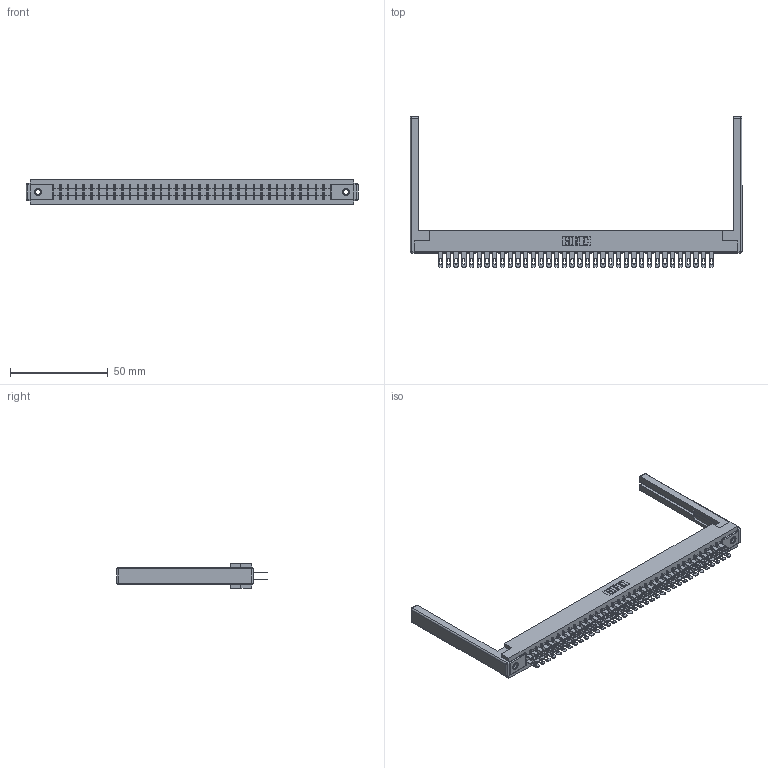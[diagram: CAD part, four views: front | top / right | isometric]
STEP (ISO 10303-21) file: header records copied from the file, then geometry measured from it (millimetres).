
FILE_DESCRIPTION (( 'STEP AP203' ), '1' );
FILE_NAME ('355-072-500-568.STEP', '2019-09-12T17:55:40', ( '' ), ( '' ), 'SwSTEP 2.0', 'SolidWorks 2016', '' );
FILE_SCHEMA (( 'CONFIG_CONTROL_DESIGN' ));
Length unit declared in the file: inch
Products named in the file (5): 307-220-068; 355-072-500-568; 305 Part_.156 Dia; 345-250-001_345-250-001-102; 305-290-001_500
Assembly tree (77 placements, depth 2):
  355-072-500-568
    305 Part_.156 Dia
    305-290-001_500  x72
    345-250-001_345-250-001-102  x2
    307-220-068  x2
Bounding box: 170.08 x 77.14 x 12.7 mm (x, y, z)
Volume: 21821.1 mm3; surface area: 28217.7 mm2
Topology: 77 solids, 77 shells, 3870 faces, 11038 edges, 7144 vertices
Faces by surface type: plane 2172, cylinder 1530, sphere 152, cone 12, torus 4
Entity records: 42490 total; most frequent: CARTESIAN_POINT 7003, ORIENTED_EDGE 6942, DIRECTION 6801, EDGE_CURVE 3471, LINE 2789, VECTOR 2789, VERTEX_POINT 2208, AXIS2_PLACEMENT_3D 2006
